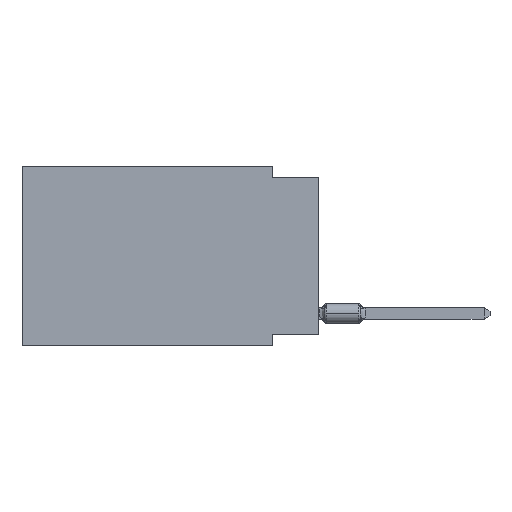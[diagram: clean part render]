
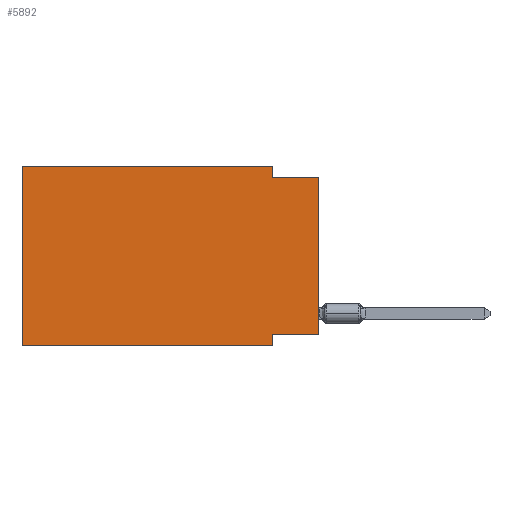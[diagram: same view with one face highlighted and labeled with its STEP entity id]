
A CAD part, left-side view. The second image highlights one B-rep face of the part: STEP entity #5892.
In plain terms, the highlighted planar face has unit normal (-1, 0, 0).
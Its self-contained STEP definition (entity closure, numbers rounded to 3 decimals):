
#46 = CARTESIAN_POINT ( 'NONE',  ( 0., 16.383, 0. ) ) ;
#157 = VECTOR ( 'NONE', #2545, 1000. ) ;
#391 = VECTOR ( 'NONE', #7574, 1000. ) ;
#464 = VERTEX_POINT ( 'NONE', #9134 ) ;
#495 = VECTOR ( 'NONE', #982, 1000. ) ;
#502 = LINE ( 'NONE', #8517, #157 ) ;
#530 = EDGE_CURVE ( 'NONE', #464, #6901, #1907, .T. ) ;
#644 = FACE_OUTER_BOUND ( 'NONE', #3119, .T. ) ;
#775 = VERTEX_POINT ( 'NONE', #2826 ) ;
#798 = LINE ( 'NONE', #8107, #2659 ) ;
#982 = DIRECTION ( 'NONE',  ( 0., 0., -1. ) ) ;
#1266 = CARTESIAN_POINT ( 'NONE',  ( 0., 16.383, 0. ) ) ;
#1710 = CARTESIAN_POINT ( 'NONE',  ( 0., 2.54, -9.271 ) ) ;
#1827 = ORIENTED_EDGE ( 'NONE', *, *, #10602, .F. ) ;
#1907 = LINE ( 'NONE', #8040, #5488 ) ;
#1910 = VECTOR ( 'NONE', #3384, 1000. ) ;
#2545 = DIRECTION ( 'NONE',  ( 0., 1., 0. ) ) ;
#2659 = VECTOR ( 'NONE', #12749, 1000. ) ;
#2812 = DIRECTION ( 'NONE',  ( 0., -1., 0. ) ) ;
#2826 = CARTESIAN_POINT ( 'NONE',  ( 0., 0., -0.635 ) ) ;
#2929 = CARTESIAN_POINT ( 'NONE',  ( 0., 0., 0. ) ) ;
#3039 = ORIENTED_EDGE ( 'NONE', *, *, #14821, .F. ) ;
#3119 = EDGE_LOOP ( 'NONE', ( #4415, #4439, #1827, #8799, #3039, #11327, #10271, #7221 ) ) ;
#3384 = DIRECTION ( 'NONE',  ( 0., 0., 1. ) ) ;
#4415 = ORIENTED_EDGE ( 'NONE', *, *, #11801, .T. ) ;
#4439 = ORIENTED_EDGE ( 'NONE', *, *, #4722, .F. ) ;
#4722 = EDGE_CURVE ( 'NONE', #6813, #775, #9118, .T. ) ;
#4740 = LINE ( 'NONE', #11892, #495 ) ;
#5185 = VERTEX_POINT ( 'NONE', #46 ) ;
#5207 = CARTESIAN_POINT ( 'NONE',  ( 0., 16.383, 0. ) ) ;
#5436 = PLANE ( 'NONE',  #10629 ) ;
#5488 = VECTOR ( 'NONE', #6850, 1000. ) ;
#5523 = EDGE_CURVE ( 'NONE', #12584, #6901, #4740, .T. ) ;
#5722 = VERTEX_POINT ( 'NONE', #13299 ) ;
#5892 = ADVANCED_FACE ( 'NONE', ( #644 ), #5436, .F. ) ;
#6277 = CARTESIAN_POINT ( 'NONE',  ( 0., 2.54, 0. ) ) ;
#6597 = CARTESIAN_POINT ( 'NONE',  ( 0., 0., -0.635 ) ) ;
#6813 = VERTEX_POINT ( 'NONE', #9617 ) ;
#6850 = DIRECTION ( 'NONE',  ( 0., -1., 0. ) ) ;
#6901 = VERTEX_POINT ( 'NONE', #13145 ) ;
#6929 = VECTOR ( 'NONE', #9049, 1000. ) ;
#7221 = ORIENTED_EDGE ( 'NONE', *, *, #14619, .F. ) ;
#7458 = CARTESIAN_POINT ( 'NONE',  ( 0., 16.383, 0. ) ) ;
#7574 = DIRECTION ( 'NONE',  ( 0., 0., 1. ) ) ;
#8040 = CARTESIAN_POINT ( 'NONE',  ( 0., 16.383, -9.906 ) ) ;
#8107 = CARTESIAN_POINT ( 'NONE',  ( 0., 2.54, 0. ) ) ;
#8517 = CARTESIAN_POINT ( 'NONE',  ( 0., 0., -9.271 ) ) ;
#8791 = LINE ( 'NONE', #7458, #9754 ) ;
#8799 = ORIENTED_EDGE ( 'NONE', *, *, #8958, .F. ) ;
#8958 = EDGE_CURVE ( 'NONE', #5185, #12557, #8791, .T. ) ;
#9049 = DIRECTION ( 'NONE',  ( 0., -1., 0. ) ) ;
#9118 = LINE ( 'NONE', #6597, #6929 ) ;
#9134 = CARTESIAN_POINT ( 'NONE',  ( 0., 16.383, -9.906 ) ) ;
#9617 = CARTESIAN_POINT ( 'NONE',  ( 0., 2.54, -0.635 ) ) ;
#9754 = VECTOR ( 'NONE', #2812, 1000. ) ;
#10241 = DIRECTION ( 'NONE',  ( 0., 0., -1. ) ) ;
#10271 = ORIENTED_EDGE ( 'NONE', *, *, #5523, .F. ) ;
#10602 = EDGE_CURVE ( 'NONE', #12557, #6813, #798, .T. ) ;
#10629 = AXIS2_PLACEMENT_3D ( 'NONE', #5207, #15101, #10241 ) ;
#11327 = ORIENTED_EDGE ( 'NONE', *, *, #530, .T. ) ;
#11801 = EDGE_CURVE ( 'NONE', #5722, #775, #13774, .T. ) ;
#11892 = CARTESIAN_POINT ( 'NONE',  ( 0., 2.54, -9.906 ) ) ;
#12038 = LINE ( 'NONE', #1266, #1910 ) ;
#12557 = VERTEX_POINT ( 'NONE', #6277 ) ;
#12584 = VERTEX_POINT ( 'NONE', #1710 ) ;
#12749 = DIRECTION ( 'NONE',  ( 0., 0., -1. ) ) ;
#13145 = CARTESIAN_POINT ( 'NONE',  ( 0., 2.54, -9.906 ) ) ;
#13299 = CARTESIAN_POINT ( 'NONE',  ( 0., 0., -9.271 ) ) ;
#13774 = LINE ( 'NONE', #2929, #391 ) ;
#14619 = EDGE_CURVE ( 'NONE', #5722, #12584, #502, .T. ) ;
#14821 = EDGE_CURVE ( 'NONE', #464, #5185, #12038, .T. ) ;
#15101 = DIRECTION ( 'NONE',  ( 1., 0., 0. ) ) ;
